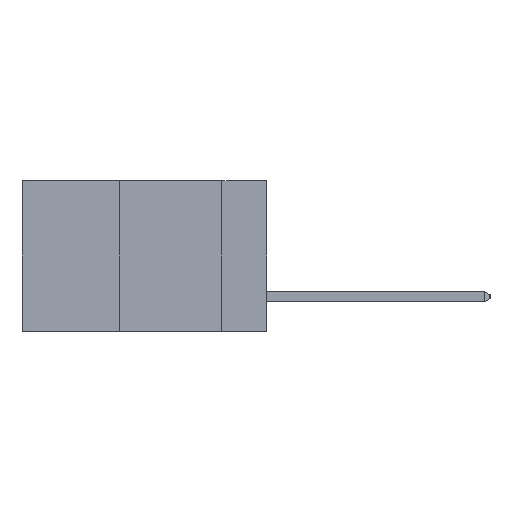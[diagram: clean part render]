
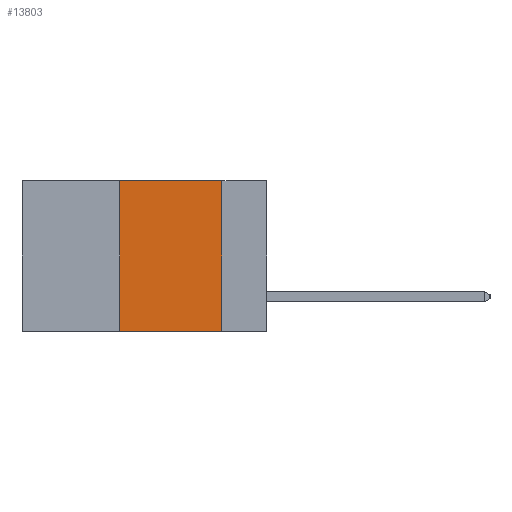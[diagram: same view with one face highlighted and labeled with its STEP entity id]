
A CAD part, left-side view. The second image highlights one B-rep face of the part: STEP entity #13803.
In plain terms, the highlighted planar face has unit normal (-1, 0, 0).
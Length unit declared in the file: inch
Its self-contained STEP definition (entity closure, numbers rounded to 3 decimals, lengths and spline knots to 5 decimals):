
#435 = CARTESIAN_POINT ( 'NONE',  ( 0., 0.11, 0. ) ) ;
#538 = LINE ( 'NONE', #542, #18474 ) ;
#542 = CARTESIAN_POINT ( 'NONE',  ( 0., 0.6, -0.37 ) ) ;
#869 = ORIENTED_EDGE ( 'NONE', *, *, #5735, .F. ) ;
#1807 = DIRECTION ( 'NONE',  ( 0., -1., 0. ) ) ;
#1933 = CARTESIAN_POINT ( 'NONE',  ( 0., 0.36, 0. ) ) ;
#3354 = VECTOR ( 'NONE', #7394, 39.37008 ) ;
#3886 = FACE_OUTER_BOUND ( 'NONE', #10706, .T. ) ;
#4118 = LINE ( 'NONE', #11269, #13562 ) ;
#4363 = LINE ( 'NONE', #8864, #3354 ) ;
#4768 = CARTESIAN_POINT ( 'NONE',  ( 0., 0.36, -0.37 ) ) ;
#4883 = ORIENTED_EDGE ( 'NONE', *, *, #9635, .T. ) ;
#5048 = DIRECTION ( 'NONE',  ( 1., 0., 0. ) ) ;
#5410 = VECTOR ( 'NONE', #1807, 39.37008 ) ;
#5686 = VERTEX_POINT ( 'NONE', #1933 ) ;
#5735 = EDGE_CURVE ( 'NONE', #5686, #13679, #11121, .T. ) ;
#6580 = ORIENTED_EDGE ( 'NONE', *, *, #14824, .F. ) ;
#6963 = DIRECTION ( 'NONE',  ( 0., 0., -1. ) ) ;
#7394 = DIRECTION ( 'NONE',  ( 0., 0., -1. ) ) ;
#8176 = DIRECTION ( 'NONE',  ( 0., 0., 1. ) ) ;
#8864 = CARTESIAN_POINT ( 'NONE',  ( 0., 0.11, 0. ) ) ;
#9109 = ORIENTED_EDGE ( 'NONE', *, *, #14239, .F. ) ;
#9635 = EDGE_CURVE ( 'NONE', #12762, #18143, #538, .T. ) ;
#10706 = EDGE_LOOP ( 'NONE', ( #6580, #869, #9109, #4883 ) ) ;
#11121 = LINE ( 'NONE', #14617, #5410 ) ;
#11269 = CARTESIAN_POINT ( 'NONE',  ( 0., 0.36, 0. ) ) ;
#11344 = PLANE ( 'NONE',  #13858 ) ;
#11811 = CARTESIAN_POINT ( 'NONE',  ( 0., 0.11, -0.37 ) ) ;
#12762 = VERTEX_POINT ( 'NONE', #4768 ) ;
#13562 = VECTOR ( 'NONE', #8176, 39.37008 ) ;
#13679 = VERTEX_POINT ( 'NONE', #435 ) ;
#13803 = ADVANCED_FACE ( 'NONE', ( #3886 ), #11344, .F. ) ;
#13858 = AXIS2_PLACEMENT_3D ( 'NONE', #14560, #5048, #6963 ) ;
#14239 = EDGE_CURVE ( 'NONE', #12762, #5686, #4118, .T. ) ;
#14560 = CARTESIAN_POINT ( 'NONE',  ( 0., 0.6, 0. ) ) ;
#14617 = CARTESIAN_POINT ( 'NONE',  ( 0., 0.6, 0. ) ) ;
#14824 = EDGE_CURVE ( 'NONE', #13679, #18143, #4363, .T. ) ;
#14998 = DIRECTION ( 'NONE',  ( 0., -1., 0. ) ) ;
#18143 = VERTEX_POINT ( 'NONE', #11811 ) ;
#18474 = VECTOR ( 'NONE', #14998, 39.37008 ) ;
